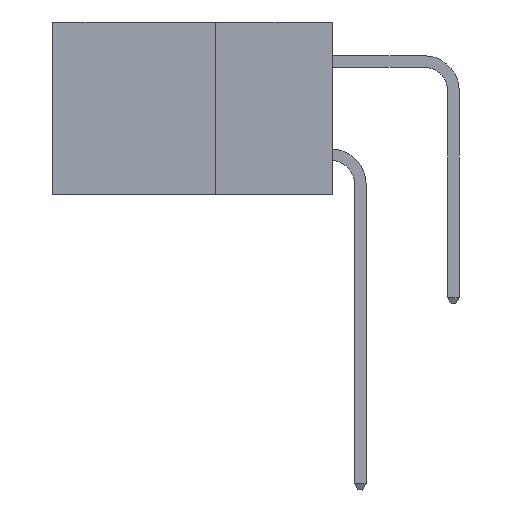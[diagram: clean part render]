
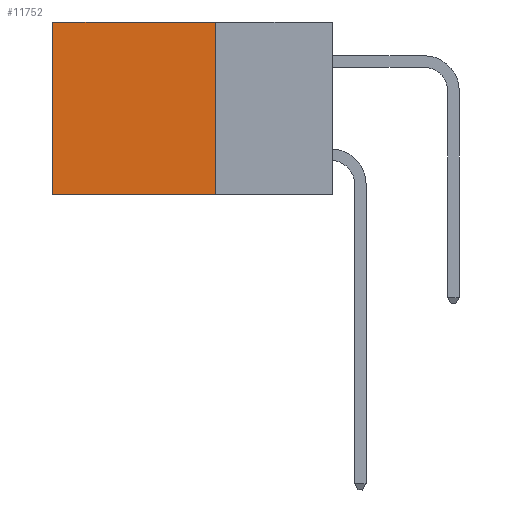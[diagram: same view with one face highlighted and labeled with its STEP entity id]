
A CAD part, left-side view. The second image highlights one B-rep face of the part: STEP entity #11752.
In plain terms, the highlighted planar face has unit normal (-1, 0, 0).
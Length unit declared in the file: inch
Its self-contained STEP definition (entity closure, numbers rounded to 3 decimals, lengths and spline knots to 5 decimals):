
#484 = CARTESIAN_POINT ( 'NONE',  ( 0.298, 0.6, 0. ) ) ;
#1237 = VERTEX_POINT ( 'NONE', #21284 ) ;
#1656 = DIRECTION ( 'NONE',  ( 0., 1., 0. ) ) ;
#2248 = LINE ( 'NONE', #484, #14147 ) ;
#2628 = DIRECTION ( 'NONE',  ( 0., 0., -1. ) ) ;
#3453 = CARTESIAN_POINT ( 'NONE',  ( 0.298, 0.25, 0. ) ) ;
#3840 = CARTESIAN_POINT ( 'NONE',  ( 0.298, 0.25, 0. ) ) ;
#5445 = DIRECTION ( 'NONE',  ( 0., 0., -1. ) ) ;
#5484 = VECTOR ( 'NONE', #8653, 39.37008 ) ;
#5736 = PLANE ( 'NONE',  #12402 ) ;
#6442 = CARTESIAN_POINT ( 'NONE',  ( 0.298, 0.25, -0.37 ) ) ;
#6775 = ORIENTED_EDGE ( 'NONE', *, *, #15250, .T. ) ;
#6954 = FACE_OUTER_BOUND ( 'NONE', #11053, .T. ) ;
#7239 = LINE ( 'NONE', #3840, #10004 ) ;
#8653 = DIRECTION ( 'NONE',  ( 0., 1., 0. ) ) ;
#9208 = VERTEX_POINT ( 'NONE', #11182 ) ;
#10004 = VECTOR ( 'NONE', #5445, 39.37008 ) ;
#10996 = ORIENTED_EDGE ( 'NONE', *, *, #13190, .T. ) ;
#11053 = EDGE_LOOP ( 'NONE', ( #6775, #23377, #24064, #10996 ) ) ;
#11179 = VECTOR ( 'NONE', #1656, 39.37008 ) ;
#11182 = CARTESIAN_POINT ( 'NONE',  ( 0.298, 0.6, -0.37 ) ) ;
#11689 = CARTESIAN_POINT ( 'NONE',  ( 0.298, 0.25, 0. ) ) ;
#11752 = ADVANCED_FACE ( 'NONE', ( #6954 ), #5736, .F. ) ;
#11850 = DIRECTION ( 'NONE',  ( 1., 0., 0. ) ) ;
#12402 = AXIS2_PLACEMENT_3D ( 'NONE', #11689, #11850, #24600 ) ;
#12441 = EDGE_CURVE ( 'NONE', #16547, #22977, #7239, .T. ) ;
#13190 = EDGE_CURVE ( 'NONE', #16547, #1237, #20291, .T. ) ;
#14147 = VECTOR ( 'NONE', #2628, 39.37008 ) ;
#15250 = EDGE_CURVE ( 'NONE', #1237, #9208, #2248, .T. ) ;
#16547 = VERTEX_POINT ( 'NONE', #3453 ) ;
#16986 = EDGE_CURVE ( 'NONE', #22977, #9208, #21690, .T. ) ;
#20291 = LINE ( 'NONE', #20837, #11179 ) ;
#20837 = CARTESIAN_POINT ( 'NONE',  ( 0.298, 0.25, 0. ) ) ;
#21284 = CARTESIAN_POINT ( 'NONE',  ( 0.298, 0.6, 0. ) ) ;
#21690 = LINE ( 'NONE', #6442, #5484 ) ;
#22977 = VERTEX_POINT ( 'NONE', #23433 ) ;
#23377 = ORIENTED_EDGE ( 'NONE', *, *, #16986, .F. ) ;
#23433 = CARTESIAN_POINT ( 'NONE',  ( 0.298, 0.25, -0.37 ) ) ;
#24064 = ORIENTED_EDGE ( 'NONE', *, *, #12441, .F. ) ;
#24600 = DIRECTION ( 'NONE',  ( 0., 0., -1. ) ) ;
